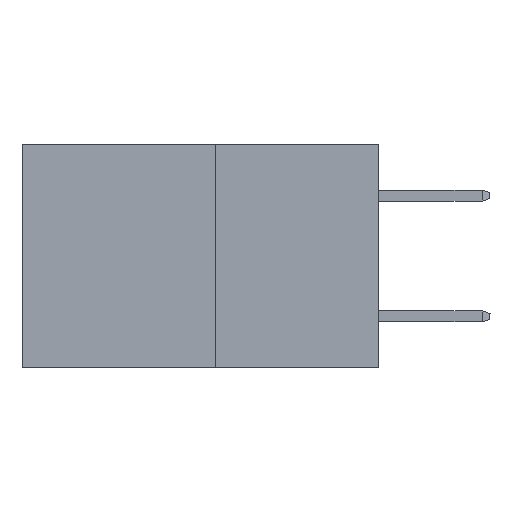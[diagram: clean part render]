
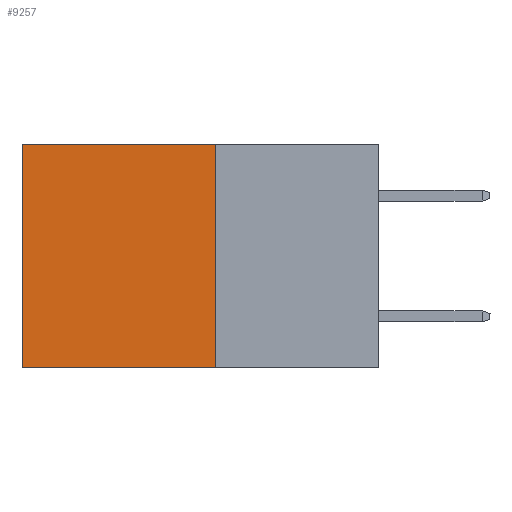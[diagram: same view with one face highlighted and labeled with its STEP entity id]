
A CAD part, left-side view. The second image highlights one B-rep face of the part: STEP entity #9257.
In plain terms, the highlighted planar face has unit normal (-1, 0, 0).
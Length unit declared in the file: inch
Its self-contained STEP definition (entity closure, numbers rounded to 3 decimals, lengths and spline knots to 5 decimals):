
#104 = DIRECTION ( 'NONE',  ( 0., 1., 0. ) ) ;
#181 = DIRECTION ( 'NONE',  ( 0., 0., -1. ) ) ;
#890 = VERTEX_POINT ( 'NONE', #6310 ) ;
#1156 = LINE ( 'NONE', #7634, #9340 ) ;
#1518 = VERTEX_POINT ( 'NONE', #4667 ) ;
#1879 = DIRECTION ( 'NONE',  ( 0., 0., -1. ) ) ;
#2351 = AXIS2_PLACEMENT_3D ( 'NONE', #9141, #5181, #181 ) ;
#2405 = ORIENTED_EDGE ( 'NONE', *, *, #4769, .T. ) ;
#2755 = EDGE_CURVE ( 'NONE', #4669, #1518, #10500, .T. ) ;
#3387 = LINE ( 'NONE', #5108, #7772 ) ;
#3743 = EDGE_LOOP ( 'NONE', ( #2405, #6738, #5995, #9157 ) ) ;
#4246 = CARTESIAN_POINT ( 'NONE',  ( 0.277, 0.27, 0. ) ) ;
#4667 = CARTESIAN_POINT ( 'NONE',  ( 0.277, 0.59, 0. ) ) ;
#4669 = VERTEX_POINT ( 'NONE', #4246 ) ;
#4769 = EDGE_CURVE ( 'NONE', #1518, #890, #1156, .T. ) ;
#5108 = CARTESIAN_POINT ( 'NONE',  ( 0.277, 0.27, -0.37 ) ) ;
#5181 = DIRECTION ( 'NONE',  ( 1., 0., 0. ) ) ;
#5783 = VERTEX_POINT ( 'NONE', #5805 ) ;
#5805 = CARTESIAN_POINT ( 'NONE',  ( 0.277, 0.27, -0.37 ) ) ;
#5901 = FACE_OUTER_BOUND ( 'NONE', #3743, .T. ) ;
#5995 = ORIENTED_EDGE ( 'NONE', *, *, #7508, .F. ) ;
#6310 = CARTESIAN_POINT ( 'NONE',  ( 0.277, 0.59, -0.37 ) ) ;
#6362 = DIRECTION ( 'NONE',  ( 0., 1., 0. ) ) ;
#6535 = CARTESIAN_POINT ( 'NONE',  ( 0.277, 0.27, 0. ) ) ;
#6738 = ORIENTED_EDGE ( 'NONE', *, *, #9204, .F. ) ;
#6752 = PLANE ( 'NONE',  #2351 ) ;
#6922 = VECTOR ( 'NONE', #9461, 39.37008 ) ;
#7074 = CARTESIAN_POINT ( 'NONE',  ( 0.277, 0.27, -0.37 ) ) ;
#7508 = EDGE_CURVE ( 'NONE', #4669, #5783, #9029, .T. ) ;
#7634 = CARTESIAN_POINT ( 'NONE',  ( 0.277, 0.59, -0.37 ) ) ;
#7772 = VECTOR ( 'NONE', #104, 39.37008 ) ;
#8174 = VECTOR ( 'NONE', #6362, 39.37008 ) ;
#9029 = LINE ( 'NONE', #7074, #6922 ) ;
#9141 = CARTESIAN_POINT ( 'NONE',  ( 0.277, 0.27, -0.37 ) ) ;
#9157 = ORIENTED_EDGE ( 'NONE', *, *, #2755, .T. ) ;
#9204 = EDGE_CURVE ( 'NONE', #5783, #890, #3387, .T. ) ;
#9257 = ADVANCED_FACE ( 'NONE', ( #5901 ), #6752, .F. ) ;
#9340 = VECTOR ( 'NONE', #1879, 39.37008 ) ;
#9461 = DIRECTION ( 'NONE',  ( 0., 0., -1. ) ) ;
#10500 = LINE ( 'NONE', #6535, #8174 ) ;
